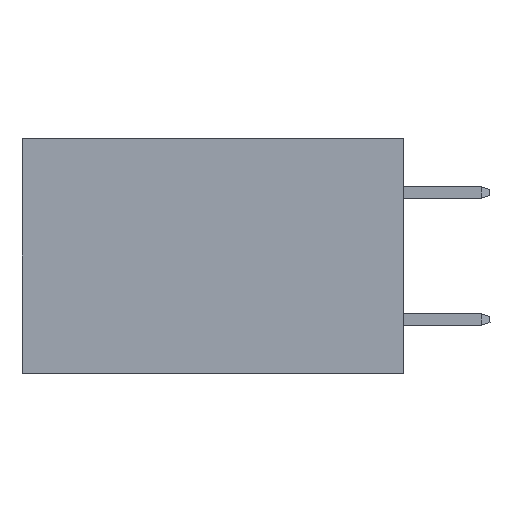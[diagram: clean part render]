
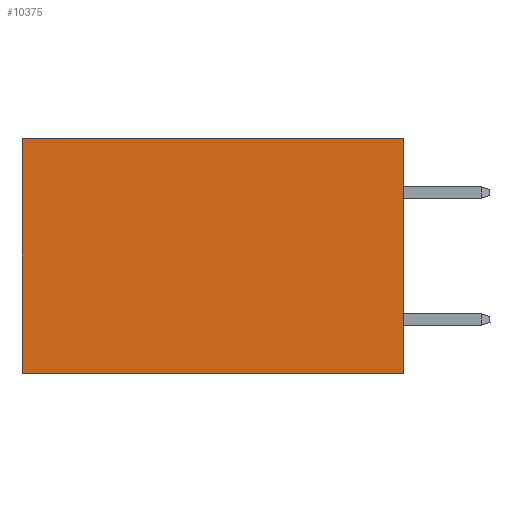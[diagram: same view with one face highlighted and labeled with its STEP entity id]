
A CAD part, left-side view. The second image highlights one B-rep face of the part: STEP entity #10375.
In plain terms, the highlighted planar face has unit normal (-1, 0, 0).
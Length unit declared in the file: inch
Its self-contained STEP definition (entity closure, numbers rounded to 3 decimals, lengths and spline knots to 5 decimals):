
#458 = VECTOR ( 'NONE', #4983, 39.37008 ) ;
#701 = VERTEX_POINT ( 'NONE', #4508 ) ;
#940 = CARTESIAN_POINT ( 'NONE',  ( 0.2875, 0., -0.37 ) ) ;
#1016 = DIRECTION ( 'NONE',  ( 0., 1., 0. ) ) ;
#1416 = CARTESIAN_POINT ( 'NONE',  ( 0.2875, 0., 0. ) ) ;
#1654 = VERTEX_POINT ( 'NONE', #13264 ) ;
#2137 = DIRECTION ( 'NONE',  ( 0., 1., 0. ) ) ;
#2209 = LINE ( 'NONE', #940, #11199 ) ;
#2415 = ORIENTED_EDGE ( 'NONE', *, *, #10105, .F. ) ;
#2575 = PLANE ( 'NONE',  #11830 ) ;
#2656 = EDGE_CURVE ( 'NONE', #4020, #4652, #10214, .T. ) ;
#2820 = EDGE_CURVE ( 'NONE', #4652, #1654, #9128, .T. ) ;
#4020 = VERTEX_POINT ( 'NONE', #1416 ) ;
#4508 = CARTESIAN_POINT ( 'NONE',  ( 0.2875, 0., -0.37 ) ) ;
#4652 = VERTEX_POINT ( 'NONE', #9172 ) ;
#4983 = DIRECTION ( 'NONE',  ( 0., 0., -1. ) ) ;
#5019 = DIRECTION ( 'NONE',  ( 1., 0., 0. ) ) ;
#5630 = EDGE_LOOP ( 'NONE', ( #11068, #9207, #2415, #11438 ) ) ;
#5860 = VECTOR ( 'NONE', #1016, 39.37008 ) ;
#6118 = CARTESIAN_POINT ( 'NONE',  ( 0.2875, 0., 0. ) ) ;
#6221 = CARTESIAN_POINT ( 'NONE',  ( 0.2875, 0., 0. ) ) ;
#8033 = LINE ( 'NONE', #6118, #458 ) ;
#8064 = DIRECTION ( 'NONE',  ( 0., 0., -1. ) ) ;
#9128 = LINE ( 'NONE', #12138, #12891 ) ;
#9172 = CARTESIAN_POINT ( 'NONE',  ( 0.2875, 0.6, 0. ) ) ;
#9207 = ORIENTED_EDGE ( 'NONE', *, *, #10494, .F. ) ;
#10005 = DIRECTION ( 'NONE',  ( 0., 0., -1. ) ) ;
#10105 = EDGE_CURVE ( 'NONE', #4020, #701, #8033, .T. ) ;
#10214 = LINE ( 'NONE', #6221, #5860 ) ;
#10375 = ADVANCED_FACE ( 'NONE', ( #12844 ), #2575, .F. ) ;
#10494 = EDGE_CURVE ( 'NONE', #701, #1654, #2209, .T. ) ;
#11068 = ORIENTED_EDGE ( 'NONE', *, *, #2820, .T. ) ;
#11199 = VECTOR ( 'NONE', #2137, 39.37008 ) ;
#11438 = ORIENTED_EDGE ( 'NONE', *, *, #2656, .T. ) ;
#11769 = CARTESIAN_POINT ( 'NONE',  ( 0.2875, 0., 0. ) ) ;
#11830 = AXIS2_PLACEMENT_3D ( 'NONE', #11769, #5019, #10005 ) ;
#12138 = CARTESIAN_POINT ( 'NONE',  ( 0.2875, 0.6, 0. ) ) ;
#12844 = FACE_OUTER_BOUND ( 'NONE', #5630, .T. ) ;
#12891 = VECTOR ( 'NONE', #8064, 39.37008 ) ;
#13264 = CARTESIAN_POINT ( 'NONE',  ( 0.2875, 0.6, -0.37 ) ) ;
